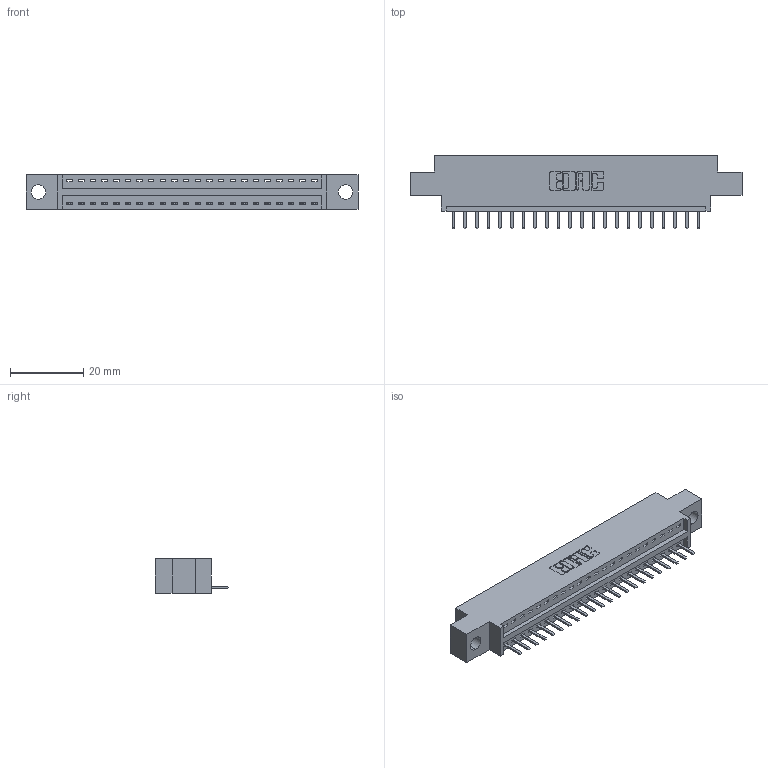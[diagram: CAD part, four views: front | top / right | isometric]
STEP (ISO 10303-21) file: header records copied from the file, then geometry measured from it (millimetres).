
FILE_DESCRIPTION (( 'STEP AP203' ), '1' );
FILE_NAME ('346-022-520-604.STEP', '2022-05-05T19:06:56', ( '' ), ( '' ), 'SwSTEP 2.0', 'SolidWorks 2020', '' );
FILE_SCHEMA (( 'CONFIG_CONTROL_DESIGN' ));
Length unit declared in the file: inch
Products named in the file (3): 345-292-001_345-293-120; 346-022-520-604; 346 Part_0.170 Offset - 0.156 Dia-TH
Assembly tree (23 placements, depth 2):
  346-022-520-604
    346 Part_0.170 Offset - 0.156 Dia-TH
    345-292-001_345-293-120  x22
Bounding box: 90.42 x 20.02 x 9.4 mm (x, y, z)
Volume: 8193.9 mm3; surface area: 9811.9 mm2
Topology: 23 solids, 23 shells, 1504 faces, 4425 edges, 2890 vertices
Faces by surface type: plane 1018, cylinder 486
Entity records: 17011 total; most frequent: CARTESIAN_POINT 2944, ORIENTED_EDGE 2886, DIRECTION 2607, EDGE_CURVE 1443, VECTOR 1219, LINE 1219, VERTEX_POINT 958, AXIS2_PLACEMENT_3D 694
